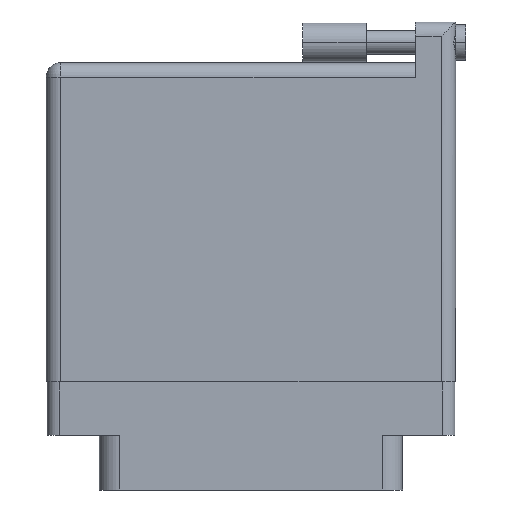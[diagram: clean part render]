
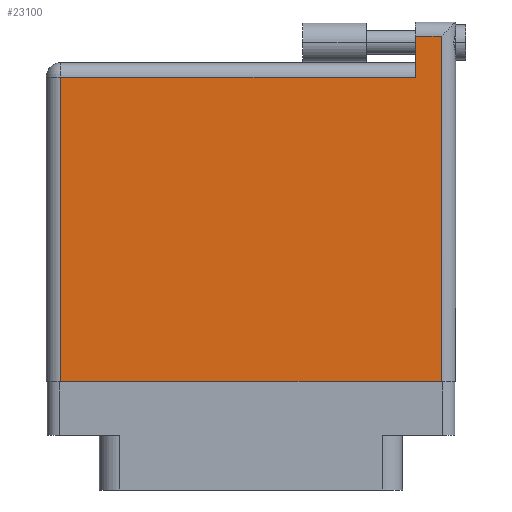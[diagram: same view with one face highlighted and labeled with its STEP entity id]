
A CAD part, front view. The second image highlights one B-rep face of the part: STEP entity #23100.
In plain terms, the highlighted face is planar.
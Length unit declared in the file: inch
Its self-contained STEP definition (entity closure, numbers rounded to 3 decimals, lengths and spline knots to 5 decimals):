
#675 = EDGE_CURVE ( 'NONE', #12310, #24264, #5034, .T. ) ;
#3713 = DIRECTION ( 'NONE',  ( 0., -1., 0. ) ) ;
#5034 = LINE ( 'NONE', #25227, #32877 ) ;
#5846 = EDGE_CURVE ( 'NONE', #24264, #8472, #15184, .T. ) ;
#6060 = DIRECTION ( 'NONE',  ( 0., -1., 0. ) ) ;
#7359 = VERTEX_POINT ( 'NONE', #14405 ) ;
#7569 = VECTOR ( 'NONE', #14142, 39.37008 ) ;
#8028 = LINE ( 'NONE', #11960, #18083 ) ;
#8472 = VERTEX_POINT ( 'NONE', #22813 ) ;
#9914 = EDGE_CURVE ( 'NONE', #34885, #23353, #13036, .T. ) ;
#10168 = LINE ( 'NONE', #26736, #32062 ) ;
#11357 = ORIENTED_EDGE ( 'NONE', *, *, #9914, .T. ) ;
#11960 = CARTESIAN_POINT ( 'NONE',  ( 0., 0., 0. ) ) ;
#12310 = VERTEX_POINT ( 'NONE', #22301 ) ;
#13036 = LINE ( 'NONE', #30073, #7569 ) ;
#13046 = ORIENTED_EDGE ( 'NONE', *, *, #5846, .T. ) ;
#13518 = CARTESIAN_POINT ( 'NONE',  ( 0., 1.566, 0. ) ) ;
#14142 = DIRECTION ( 'NONE',  ( 0., 1., 0. ) ) ;
#14405 = CARTESIAN_POINT ( 'NONE',  ( 1.811, 1.696, 0. ) ) ;
#15184 = LINE ( 'NONE', #29968, #29127 ) ;
#15961 = PLANE ( 'NONE',  #24026 ) ;
#16307 = DIRECTION ( 'NONE',  ( -1., 0., 0. ) ) ;
#16975 = CARTESIAN_POINT ( 'NONE',  ( 1.811, 1.766, 0. ) ) ;
#17008 = EDGE_CURVE ( 'NONE', #7359, #12310, #30873, .T. ) ;
#17628 = ORIENTED_EDGE ( 'NONE', *, *, #17008, .T. ) ;
#18083 = VECTOR ( 'NONE', #23553, 39.37008 ) ;
#20366 = EDGE_LOOP ( 'NONE', ( #30645, #11357, #23356, #17628, #20918, #13046 ) ) ;
#20918 = ORIENTED_EDGE ( 'NONE', *, *, #675, .T. ) ;
#22200 = EDGE_CURVE ( 'NONE', #8472, #34885, #8028, .T. ) ;
#22301 = CARTESIAN_POINT ( 'NONE',  ( 1.811, 1.496, 0. ) ) ;
#22537 = CARTESIAN_POINT ( 'NONE',  ( 0.07, 1.496, 0. ) ) ;
#22659 = CARTESIAN_POINT ( 'NONE',  ( 1.938, 1.696, 0. ) ) ;
#22813 = CARTESIAN_POINT ( 'NONE',  ( 0.07, 0., 0. ) ) ;
#23100 = ADVANCED_FACE ( 'NONE', ( #28994 ), #15961, .F. ) ;
#23353 = VERTEX_POINT ( 'NONE', #22659 ) ;
#23356 = ORIENTED_EDGE ( 'NONE', *, *, #30986, .T. ) ;
#23553 = DIRECTION ( 'NONE',  ( 1., 0., 0. ) ) ;
#24026 = AXIS2_PLACEMENT_3D ( 'NONE', #13518, #26696, #16307 ) ;
#24264 = VERTEX_POINT ( 'NONE', #22537 ) ;
#24520 = CARTESIAN_POINT ( 'NONE',  ( 1.938, 0., 0. ) ) ;
#24998 = DIRECTION ( 'NONE',  ( -1., 0., 0. ) ) ;
#25227 = CARTESIAN_POINT ( 'NONE',  ( 0., 1.496, 0. ) ) ;
#26203 = VECTOR ( 'NONE', #3713, 39.37008 ) ;
#26696 = DIRECTION ( 'NONE',  ( 0., 0., -1. ) ) ;
#26736 = CARTESIAN_POINT ( 'NONE',  ( 0., 1.696, 0. ) ) ;
#28994 = FACE_OUTER_BOUND ( 'NONE', #20366, .T. ) ;
#29127 = VECTOR ( 'NONE', #6060, 39.37008 ) ;
#29555 = DIRECTION ( 'NONE',  ( -1., 0., 0. ) ) ;
#29968 = CARTESIAN_POINT ( 'NONE',  ( 0.07, 0., 0. ) ) ;
#30073 = CARTESIAN_POINT ( 'NONE',  ( 1.938, 1.766, 0. ) ) ;
#30645 = ORIENTED_EDGE ( 'NONE', *, *, #22200, .T. ) ;
#30873 = LINE ( 'NONE', #16975, #26203 ) ;
#30986 = EDGE_CURVE ( 'NONE', #23353, #7359, #10168, .T. ) ;
#32062 = VECTOR ( 'NONE', #29555, 39.37008 ) ;
#32877 = VECTOR ( 'NONE', #24998, 39.37008 ) ;
#34885 = VERTEX_POINT ( 'NONE', #24520 ) ;
